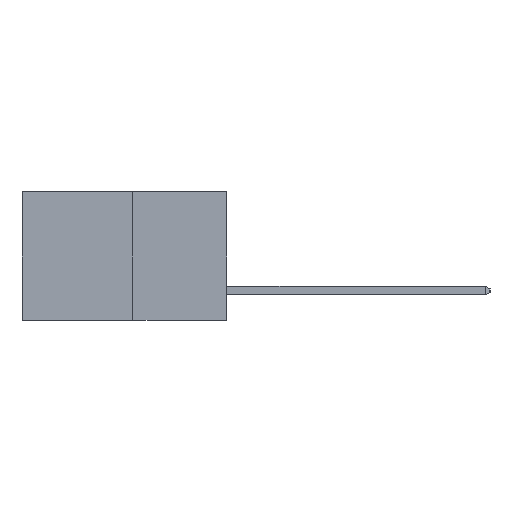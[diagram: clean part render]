
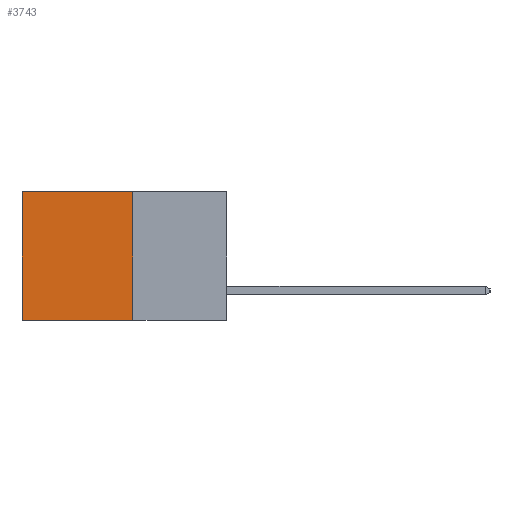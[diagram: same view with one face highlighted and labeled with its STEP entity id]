
A CAD part, left-side view. The second image highlights one B-rep face of the part: STEP entity #3743.
In plain terms, the highlighted planar face has unit normal (-1, 0, 0).
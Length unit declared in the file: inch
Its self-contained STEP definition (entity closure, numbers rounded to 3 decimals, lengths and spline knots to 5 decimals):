
#1297 = VERTEX_POINT ( 'NONE', #16868 ) ;
#1704 = VECTOR ( 'NONE', #14154, 39.37008 ) ;
#1999 = CARTESIAN_POINT ( 'NONE',  ( 0.277, 0.59, -0.37 ) ) ;
#2792 = ORIENTED_EDGE ( 'NONE', *, *, #4764, .T. ) ;
#3743 = ADVANCED_FACE ( 'NONE', ( #18526 ), #21199, .F. ) ;
#4197 = DIRECTION ( 'NONE',  ( 0., 0., -1. ) ) ;
#4764 = EDGE_CURVE ( 'NONE', #7654, #7254, #4902, .T. ) ;
#4902 = LINE ( 'NONE', #8232, #9352 ) ;
#5579 = ORIENTED_EDGE ( 'NONE', *, *, #13811, .F. ) ;
#5856 = CARTESIAN_POINT ( 'NONE',  ( 0.277, 0.27, -0.37 ) ) ;
#6520 = CARTESIAN_POINT ( 'NONE',  ( 0.277, 0.27, -0.37 ) ) ;
#6715 = ORIENTED_EDGE ( 'NONE', *, *, #15173, .T. ) ;
#6832 = CARTESIAN_POINT ( 'NONE',  ( 0.277, 0.59, 0. ) ) ;
#7252 = VECTOR ( 'NONE', #4197, 39.37008 ) ;
#7254 = VERTEX_POINT ( 'NONE', #1999 ) ;
#7564 = CARTESIAN_POINT ( 'NONE',  ( 0.277, 0.27, 0. ) ) ;
#7654 = VERTEX_POINT ( 'NONE', #6832 ) ;
#8232 = CARTESIAN_POINT ( 'NONE',  ( 0.277, 0.59, -0.37 ) ) ;
#9087 = DIRECTION ( 'NONE',  ( 0., 1., 0. ) ) ;
#9184 = AXIS2_PLACEMENT_3D ( 'NONE', #20737, #21217, #21224 ) ;
#9352 = VECTOR ( 'NONE', #11843, 39.37008 ) ;
#10383 = ORIENTED_EDGE ( 'NONE', *, *, #11041, .F. ) ;
#10580 = LINE ( 'NONE', #7564, #1704 ) ;
#11041 = EDGE_CURVE ( 'NONE', #17737, #7254, #15703, .T. ) ;
#11279 = VECTOR ( 'NONE', #9087, 39.37008 ) ;
#11626 = LINE ( 'NONE', #5856, #7252 ) ;
#11843 = DIRECTION ( 'NONE',  ( 0., 0., -1. ) ) ;
#13811 = EDGE_CURVE ( 'NONE', #1297, #17737, #11626, .T. ) ;
#14154 = DIRECTION ( 'NONE',  ( 0., 1., 0. ) ) ;
#15173 = EDGE_CURVE ( 'NONE', #1297, #7654, #10580, .T. ) ;
#15703 = LINE ( 'NONE', #20702, #11279 ) ;
#15828 = EDGE_LOOP ( 'NONE', ( #2792, #10383, #5579, #6715 ) ) ;
#16868 = CARTESIAN_POINT ( 'NONE',  ( 0.277, 0.27, 0. ) ) ;
#17737 = VERTEX_POINT ( 'NONE', #6520 ) ;
#18526 = FACE_OUTER_BOUND ( 'NONE', #15828, .T. ) ;
#20702 = CARTESIAN_POINT ( 'NONE',  ( 0.277, 0.27, -0.37 ) ) ;
#20737 = CARTESIAN_POINT ( 'NONE',  ( 0.277, 0.27, -0.37 ) ) ;
#21199 = PLANE ( 'NONE',  #9184 ) ;
#21217 = DIRECTION ( 'NONE',  ( 1., 0., 0. ) ) ;
#21224 = DIRECTION ( 'NONE',  ( 0., 0., -1. ) ) ;
